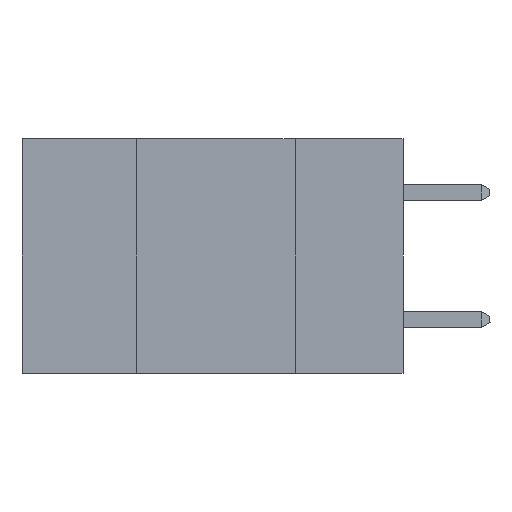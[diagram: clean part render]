
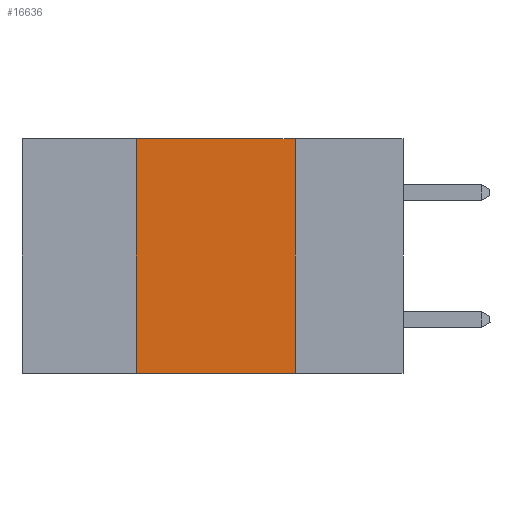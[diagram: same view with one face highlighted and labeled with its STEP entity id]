
A CAD part, left-side view. The second image highlights one B-rep face of the part: STEP entity #16636.
In plain terms, the highlighted planar face has unit normal (-1, 0, 0).
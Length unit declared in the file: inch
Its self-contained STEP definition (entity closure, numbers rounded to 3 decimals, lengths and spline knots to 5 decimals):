
#113 = LINE ( 'NONE', #16363, #13590 ) ;
#211 = EDGE_CURVE ( 'NONE', #7501, #10393, #19221, .T. ) ;
#569 = CARTESIAN_POINT ( 'NONE',  ( 0., 0.42, 0. ) ) ;
#580 = VERTEX_POINT ( 'NONE', #19960 ) ;
#2517 = ORIENTED_EDGE ( 'NONE', *, *, #9788, .F. ) ;
#3188 = ORIENTED_EDGE ( 'NONE', *, *, #11915, .F. ) ;
#4022 = FACE_OUTER_BOUND ( 'NONE', #15428, .T. ) ;
#4539 = VECTOR ( 'NONE', #6799, 39.37008 ) ;
#4860 = VECTOR ( 'NONE', #6137, 39.37008 ) ;
#5558 = CARTESIAN_POINT ( 'NONE',  ( 0., 0.17, 0. ) ) ;
#6137 = DIRECTION ( 'NONE',  ( 0., -1., 0. ) ) ;
#6711 = PLANE ( 'NONE',  #13630 ) ;
#6799 = DIRECTION ( 'NONE',  ( 0., -1., 0. ) ) ;
#7501 = VERTEX_POINT ( 'NONE', #21202 ) ;
#7726 = DIRECTION ( 'NONE',  ( 0., 0., -1. ) ) ;
#8094 = DIRECTION ( 'NONE',  ( 0., 0., 1. ) ) ;
#8477 = CARTESIAN_POINT ( 'NONE',  ( 0., 0.6, 0. ) ) ;
#9199 = LINE ( 'NONE', #15438, #4539 ) ;
#9788 = EDGE_CURVE ( 'NONE', #12138, #580, #113, .T. ) ;
#10236 = DIRECTION ( 'NONE',  ( 0., 0., -1. ) ) ;
#10393 = VERTEX_POINT ( 'NONE', #569 ) ;
#11327 = CARTESIAN_POINT ( 'NONE',  ( 0., 0.6, -0.37 ) ) ;
#11915 = EDGE_CURVE ( 'NONE', #10393, #12138, #9199, .T. ) ;
#12138 = VERTEX_POINT ( 'NONE', #5558 ) ;
#12414 = ORIENTED_EDGE ( 'NONE', *, *, #211, .F. ) ;
#12806 = ORIENTED_EDGE ( 'NONE', *, *, #21394, .T. ) ;
#13590 = VECTOR ( 'NONE', #7726, 39.37008 ) ;
#13630 = AXIS2_PLACEMENT_3D ( 'NONE', #8477, #20582, #10236 ) ;
#13986 = CARTESIAN_POINT ( 'NONE',  ( 0., 0.42, 0. ) ) ;
#14009 = VECTOR ( 'NONE', #8094, 39.37008 ) ;
#15201 = LINE ( 'NONE', #11327, #4860 ) ;
#15428 = EDGE_LOOP ( 'NONE', ( #2517, #3188, #12414, #12806 ) ) ;
#15438 = CARTESIAN_POINT ( 'NONE',  ( 0., 0.6, 0. ) ) ;
#16363 = CARTESIAN_POINT ( 'NONE',  ( 0., 0.17, 0. ) ) ;
#16636 = ADVANCED_FACE ( 'NONE', ( #4022 ), #6711, .F. ) ;
#19221 = LINE ( 'NONE', #13986, #14009 ) ;
#19960 = CARTESIAN_POINT ( 'NONE',  ( 0., 0.17, -0.37 ) ) ;
#20582 = DIRECTION ( 'NONE',  ( 1., 0., 0. ) ) ;
#21202 = CARTESIAN_POINT ( 'NONE',  ( 0., 0.42, -0.37 ) ) ;
#21394 = EDGE_CURVE ( 'NONE', #7501, #580, #15201, .T. ) ;
